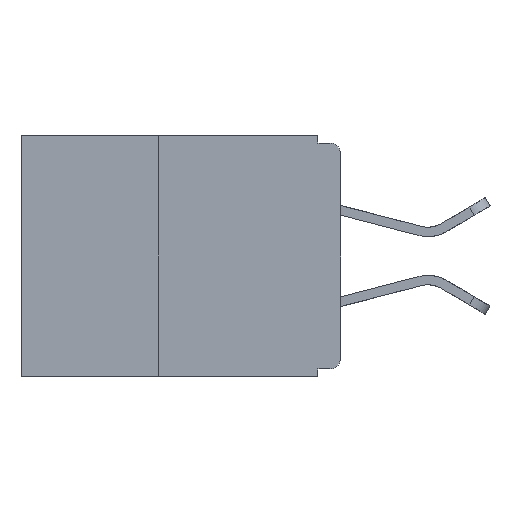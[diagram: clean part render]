
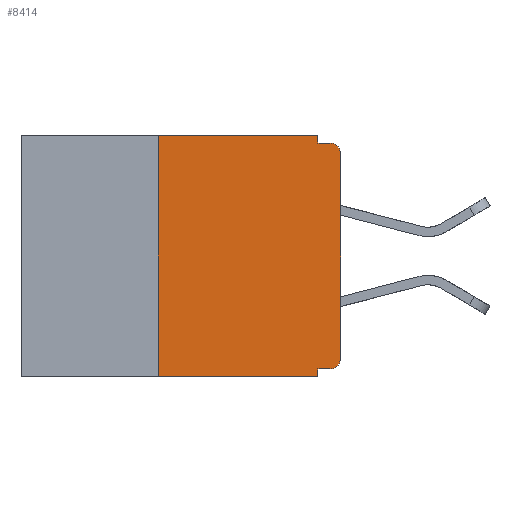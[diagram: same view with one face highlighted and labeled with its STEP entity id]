
A CAD part, left-side view. The second image highlights one B-rep face of the part: STEP entity #8414.
In plain terms, the highlighted planar face has unit normal (-1, 0, 0).
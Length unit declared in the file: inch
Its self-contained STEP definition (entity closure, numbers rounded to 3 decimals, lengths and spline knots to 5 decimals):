
#970 = VERTEX_POINT ( 'NONE', #10134 ) ;
#1034 = AXIS2_PLACEMENT_3D ( 'NONE', #25140, #15644, #1363 ) ;
#1309 = ORIENTED_EDGE ( 'NONE', *, *, #20029, .F. ) ;
#1363 = DIRECTION ( 'NONE',  ( 0., 0., -1. ) ) ;
#1368 = CARTESIAN_POINT ( 'NONE',  ( 0., 0.015, -0.305 ) ) ;
#2465 = ORIENTED_EDGE ( 'NONE', *, *, #10182, .T. ) ;
#2470 = CARTESIAN_POINT ( 'NONE',  ( 0., 0., -0.32 ) ) ;
#2779 = CARTESIAN_POINT ( 'NONE',  ( 0., 0., -0.01 ) ) ;
#2979 = EDGE_CURVE ( 'NONE', #27424, #10865, #5834, .T. ) ;
#3241 = EDGE_LOOP ( 'NONE', ( #3337, #17511, #1309, #11289, #15690, #26647, #15329, #27666, #24277, #2465 ) ) ;
#3337 = ORIENTED_EDGE ( 'NONE', *, *, #16953, .T. ) ;
#3647 = PLANE ( 'NONE',  #1034 ) ;
#3754 = DIRECTION ( 'NONE',  ( 0., 0., -1. ) ) ;
#4202 = EDGE_CURVE ( 'NONE', #970, #27424, #10188, .T. ) ;
#5834 = LINE ( 'NONE', #7364, #30389 ) ;
#6800 = EDGE_CURVE ( 'NONE', #10865, #15574, #23921, .T. ) ;
#7106 = VERTEX_POINT ( 'NONE', #9795 ) ;
#7186 = DIRECTION ( 'NONE',  ( 0., 1., 0. ) ) ;
#7364 = CARTESIAN_POINT ( 'NONE',  ( 0., 0.437, 0. ) ) ;
#7507 = VECTOR ( 'NONE', #17081, 39.37008 ) ;
#7896 = DIRECTION ( 'NONE',  ( 0., -1., 0. ) ) ;
#8414 = ADVANCED_FACE ( 'NONE', ( #9799 ), #3647, .F. ) ;
#9795 = CARTESIAN_POINT ( 'NONE',  ( 0., 0., -0.305 ) ) ;
#9799 = FACE_OUTER_BOUND ( 'NONE', #3241, .T. ) ;
#10134 = CARTESIAN_POINT ( 'NONE',  ( 0., 0.25, -0.33 ) ) ;
#10182 = EDGE_CURVE ( 'NONE', #21817, #7106, #30186, .T. ) ;
#10188 = LINE ( 'NONE', #19110, #27746 ) ;
#10486 = EDGE_CURVE ( 'NONE', #30394, #18189, #28326, .T. ) ;
#10487 = VECTOR ( 'NONE', #13945, 39.37008 ) ;
#10581 = VECTOR ( 'NONE', #13316, 39.37008 ) ;
#10865 = VERTEX_POINT ( 'NONE', #29835 ) ;
#10887 = CARTESIAN_POINT ( 'NONE',  ( 0., 0.031, -0.01 ) ) ;
#10917 = CARTESIAN_POINT ( 'NONE',  ( 0., 0., 0. ) ) ;
#11051 = VERTEX_POINT ( 'NONE', #21115 ) ;
#11079 = VERTEX_POINT ( 'NONE', #23615 ) ;
#11289 = ORIENTED_EDGE ( 'NONE', *, *, #6800, .F. ) ;
#11675 = CARTESIAN_POINT ( 'NONE',  ( 0., 0., -0.025 ) ) ;
#11904 = CARTESIAN_POINT ( 'NONE',  ( 0., 0.015, -0.32 ) ) ;
#12031 = DIRECTION ( 'NONE',  ( -1., 0., 0. ) ) ;
#13316 = DIRECTION ( 'NONE',  ( 0., 0., 1. ) ) ;
#13552 = CARTESIAN_POINT ( 'NONE',  ( 0., 0.437, -0.33 ) ) ;
#13945 = DIRECTION ( 'NONE',  ( 0., 0., -1. ) ) ;
#14839 = CARTESIAN_POINT ( 'NONE',  ( 0., 0.031, 0. ) ) ;
#15044 = AXIS2_PLACEMENT_3D ( 'NONE', #1368, #18056, #3754 ) ;
#15300 = VECTOR ( 'NONE', #7186, 39.37008 ) ;
#15329 = ORIENTED_EDGE ( 'NONE', *, *, #24653, .T. ) ;
#15570 = DIRECTION ( 'NONE',  ( 0., 0., -1. ) ) ;
#15573 = CARTESIAN_POINT ( 'NONE',  ( 0., 0.015, -0.01 ) ) ;
#15574 = VERTEX_POINT ( 'NONE', #10887 ) ;
#15644 = DIRECTION ( 'NONE',  ( 1., 0., 0. ) ) ;
#15690 = ORIENTED_EDGE ( 'NONE', *, *, #2979, .F. ) ;
#16884 = LINE ( 'NONE', #25756, #10487 ) ;
#16953 = EDGE_CURVE ( 'NONE', #7106, #30394, #28880, .T. ) ;
#17081 = DIRECTION ( 'NONE',  ( 0., -1., 0. ) ) ;
#17511 = ORIENTED_EDGE ( 'NONE', *, *, #10486, .T. ) ;
#18056 = DIRECTION ( 'NONE',  ( -1., 0., 0. ) ) ;
#18189 = VERTEX_POINT ( 'NONE', #15573 ) ;
#18309 = VECTOR ( 'NONE', #15570, 39.37008 ) ;
#18702 = CARTESIAN_POINT ( 'NONE',  ( 0., 0.25, 0. ) ) ;
#18900 = EDGE_CURVE ( 'NONE', #11079, #11051, #16884, .T. ) ;
#18934 = DIRECTION ( 'NONE',  ( 0., 0., 1. ) ) ;
#19110 = CARTESIAN_POINT ( 'NONE',  ( 0., 0.25, -0.33 ) ) ;
#19297 = AXIS2_PLACEMENT_3D ( 'NONE', #26376, #12031, #28747 ) ;
#19920 = EDGE_CURVE ( 'NONE', #21817, #11079, #23194, .T. ) ;
#20029 = EDGE_CURVE ( 'NONE', #15574, #18189, #25017, .T. ) ;
#21115 = CARTESIAN_POINT ( 'NONE',  ( 0., 0.031, -0.33 ) ) ;
#21817 = VERTEX_POINT ( 'NONE', #11904 ) ;
#22992 = LINE ( 'NONE', #13552, #23749 ) ;
#23194 = LINE ( 'NONE', #2470, #15300 ) ;
#23615 = CARTESIAN_POINT ( 'NONE',  ( 0., 0.031, -0.32 ) ) ;
#23749 = VECTOR ( 'NONE', #25580, 39.37008 ) ;
#23921 = LINE ( 'NONE', #14839, #18309 ) ;
#24277 = ORIENTED_EDGE ( 'NONE', *, *, #19920, .F. ) ;
#24653 = EDGE_CURVE ( 'NONE', #970, #11051, #22992, .T. ) ;
#25017 = LINE ( 'NONE', #2779, #7507 ) ;
#25140 = CARTESIAN_POINT ( 'NONE',  ( 0., 0.437, 0. ) ) ;
#25580 = DIRECTION ( 'NONE',  ( 0., -1., 0. ) ) ;
#25756 = CARTESIAN_POINT ( 'NONE',  ( 0., 0.031, -0.33 ) ) ;
#26376 = CARTESIAN_POINT ( 'NONE',  ( 0., 0.015, -0.025 ) ) ;
#26647 = ORIENTED_EDGE ( 'NONE', *, *, #4202, .F. ) ;
#27424 = VERTEX_POINT ( 'NONE', #18702 ) ;
#27666 = ORIENTED_EDGE ( 'NONE', *, *, #18900, .F. ) ;
#27746 = VECTOR ( 'NONE', #18934, 39.37008 ) ;
#28326 = CIRCLE ( 'NONE', #19297, 0.015 ) ;
#28747 = DIRECTION ( 'NONE',  ( 0., 0., -1. ) ) ;
#28880 = LINE ( 'NONE', #10917, #10581 ) ;
#29835 = CARTESIAN_POINT ( 'NONE',  ( 0., 0.031, 0. ) ) ;
#30186 = CIRCLE ( 'NONE', #15044, 0.015 ) ;
#30389 = VECTOR ( 'NONE', #7896, 39.37008 ) ;
#30394 = VERTEX_POINT ( 'NONE', #11675 ) ;
